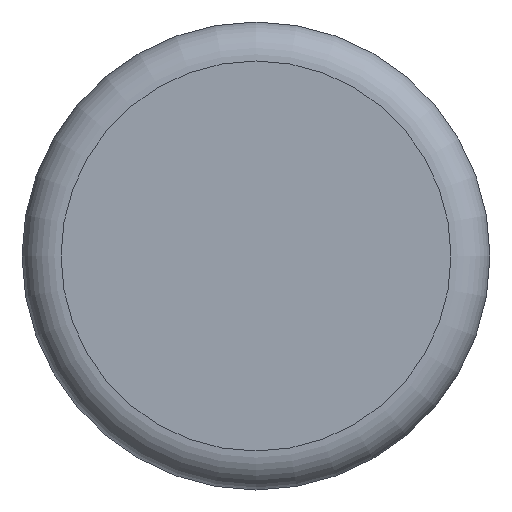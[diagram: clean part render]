
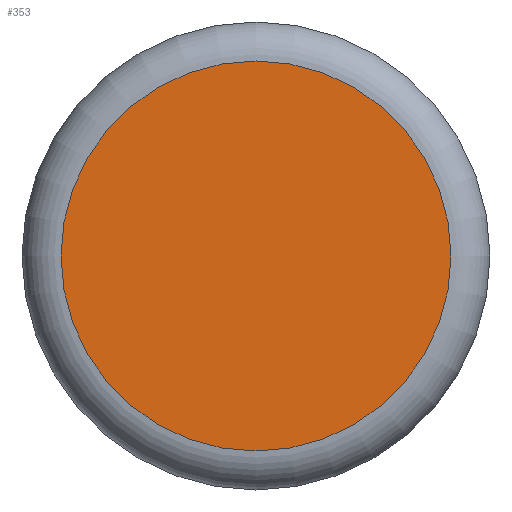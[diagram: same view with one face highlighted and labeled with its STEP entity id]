
A CAD part, front view. The second image highlights one B-rep face of the part: STEP entity #353.
In plain terms, the highlighted planar face has unit normal (0, -1, 0).
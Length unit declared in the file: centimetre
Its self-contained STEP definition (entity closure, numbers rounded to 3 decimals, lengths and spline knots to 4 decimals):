
#69=PLANE($,#381);
#94=FACE_OUTER_BOUND($,#118,.T.);
#118=EDGE_LOOP($,(#248));
#140=CIRCLE($,#377,0.5);
#156=VERTEX_POINT($,#538);
#192=EDGE_CURVE($,#156,#156,#140,.T.);
#248=ORIENTED_EDGE($,*,*,#192,.F.);
#353=ADVANCED_FACE($,(#94),#69,.T.);
#377=AXIS2_PLACEMENT_3D($,#539,#426,#427);
#381=AXIS2_PLACEMENT_3D($,#545,#434,#435);
#426=DIRECTION('center_axis',(0.,1.,0.));
#427=DIRECTION('ref_axis',(0.,0.,-1.));
#434=DIRECTION('center_axis',(0.,-1.,0.));
#435=DIRECTION('ref_axis',(0.,0.,-1.));
#538=CARTESIAN_POINT('',(0.,-4.4,0.5));
#539=CARTESIAN_POINT('Origin',(0.,-4.4,0.));
#545=CARTESIAN_POINT('Origin',(0.,-4.4,0.));
